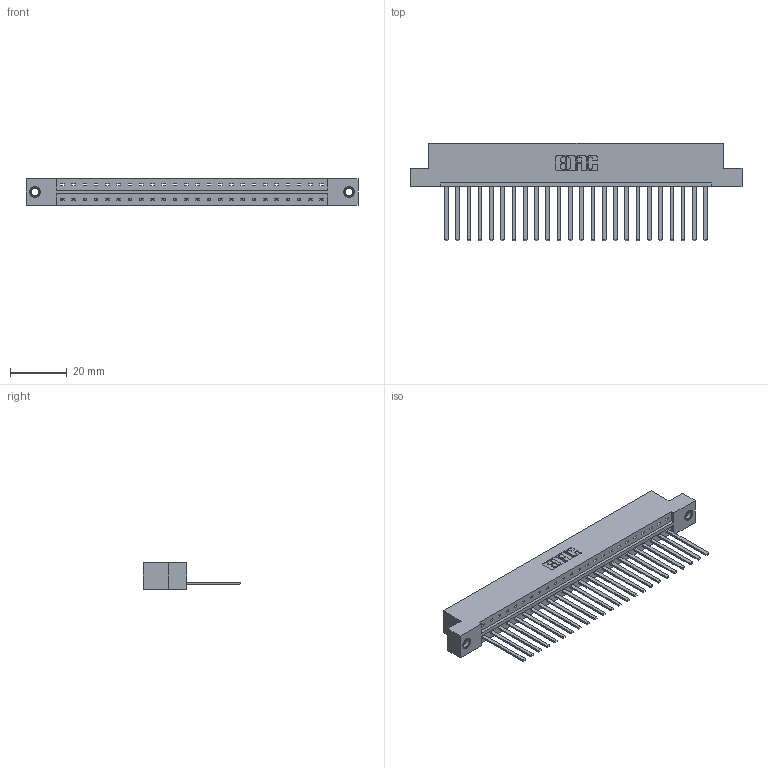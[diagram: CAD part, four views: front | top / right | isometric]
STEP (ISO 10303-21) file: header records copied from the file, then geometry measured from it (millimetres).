
FILE_DESCRIPTION (( 'STEP AP203' ), '1' );
FILE_NAME ('833-024-544-107.STEP', '2020-06-01T21:53:01', ( '' ), ( '' ), 'SwSTEP 2.0', 'SolidWorks 2020', '' );
FILE_SCHEMA (( 'CONFIG_CONTROL_DESIGN' ));
Length unit declared in the file: inch
Products named in the file (4): 833 Part_Flush - .156 Dia - TI; 833-024-544-107; 345-292-001_345-293-144; 345-250-001_345-250-005-103
Assembly tree (27 placements, depth 2):
  833-024-544-107
    833 Part_Flush - .156 Dia - TI
    345-292-001_345-293-144  x24
    345-250-001_345-250-005-103  x2
Bounding box: 116.64 x 34.3 x 9.4 mm (x, y, z)
Volume: 11846.6 mm3; surface area: 13641.3 mm2
Topology: 27 solids, 27 shells, 1422 faces, 4239 edges, 2786 vertices
Faces by surface type: plane 1014, cylinder 392, cone 12, torus 4
Entity records: 18002 total; most frequent: CARTESIAN_POINT 3089, ORIENTED_EDGE 3042, DIRECTION 2671, EDGE_CURVE 1521, LINE 1377, VECTOR 1377, VERTEX_POINT 1008, AXIS2_PLACEMENT_3D 647
